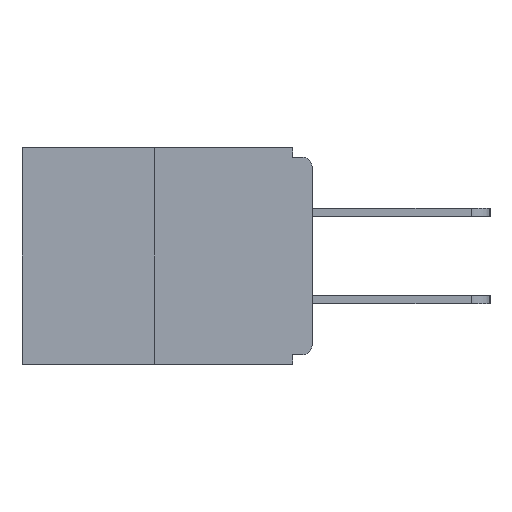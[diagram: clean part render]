
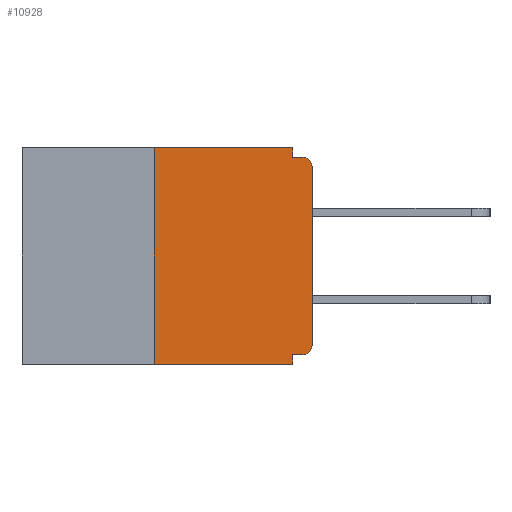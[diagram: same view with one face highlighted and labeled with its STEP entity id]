
A CAD part, left-side view. The second image highlights one B-rep face of the part: STEP entity #10928.
In plain terms, the highlighted planar face has unit normal (-1, 0, 0).
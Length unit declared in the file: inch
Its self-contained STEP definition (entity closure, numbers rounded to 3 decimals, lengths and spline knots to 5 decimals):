
#131 = EDGE_CURVE ( 'NONE', #7496, #12693, #7042, .T. ) ;
#219 = EDGE_CURVE ( 'NONE', #6645, #11678, #10148, .T. ) ;
#316 = CARTESIAN_POINT ( 'NONE',  ( 0., 0.46, 0. ) ) ;
#330 = CIRCLE ( 'NONE', #7711, 0.015 ) ;
#387 = CARTESIAN_POINT ( 'NONE',  ( 0., 0.031, -0.343 ) ) ;
#524 = PLANE ( 'NONE',  #10026 ) ;
#938 = ORIENTED_EDGE ( 'NONE', *, *, #5885, .T. ) ;
#1329 = LINE ( 'NONE', #316, #9888 ) ;
#1648 = CARTESIAN_POINT ( 'NONE',  ( 0., 0.25, 0. ) ) ;
#1830 = CARTESIAN_POINT ( 'NONE',  ( 0., 0.25, -0.343 ) ) ;
#2160 = VERTEX_POINT ( 'NONE', #387 ) ;
#2193 = DIRECTION ( 'NONE',  ( -1., 0., 0. ) ) ;
#2514 = AXIS2_PLACEMENT_3D ( 'NONE', #9028, #10268, #6293 ) ;
#2884 = VECTOR ( 'NONE', #3834, 39.37008 ) ;
#3396 = DIRECTION ( 'NONE',  ( 0., -1., 0. ) ) ;
#3625 = CARTESIAN_POINT ( 'NONE',  ( 0., 0.25, 0. ) ) ;
#3639 = EDGE_CURVE ( 'NONE', #6916, #2160, #11748, .T. ) ;
#3834 = DIRECTION ( 'NONE',  ( 0., 0., -1. ) ) ;
#3948 = VERTEX_POINT ( 'NONE', #9258 ) ;
#3983 = CARTESIAN_POINT ( 'NONE',  ( 0., 0.015, -0.328 ) ) ;
#4005 = ORIENTED_EDGE ( 'NONE', *, *, #7809, .T. ) ;
#4023 = CIRCLE ( 'NONE', #2514, 0.015 ) ;
#4101 = CARTESIAN_POINT ( 'NONE',  ( 0., 0., -0.328 ) ) ;
#4320 = CARTESIAN_POINT ( 'NONE',  ( 0., 0., -0.015 ) ) ;
#4569 = LINE ( 'NONE', #11820, #2884 ) ;
#4978 = EDGE_CURVE ( 'NONE', #11678, #2160, #4569, .T. ) ;
#5020 = DIRECTION ( 'NONE',  ( 0., 1., 0. ) ) ;
#5159 = VERTEX_POINT ( 'NONE', #3625 ) ;
#5363 = CARTESIAN_POINT ( 'NONE',  ( 0., 0.031, 0. ) ) ;
#5516 = DIRECTION ( 'NONE',  ( 1., 0., 0. ) ) ;
#5885 = EDGE_CURVE ( 'NONE', #3948, #9694, #330, .T. ) ;
#6252 = CARTESIAN_POINT ( 'NONE',  ( 0., 0.031, -0.328 ) ) ;
#6293 = DIRECTION ( 'NONE',  ( 0., 0., -1. ) ) ;
#6373 = CARTESIAN_POINT ( 'NONE',  ( 0., 0.031, 0. ) ) ;
#6432 = ORIENTED_EDGE ( 'NONE', *, *, #7724, .T. ) ;
#6645 = VERTEX_POINT ( 'NONE', #3983 ) ;
#6748 = LINE ( 'NONE', #4320, #11732 ) ;
#6855 = VECTOR ( 'NONE', #5020, 39.37008 ) ;
#6916 = VERTEX_POINT ( 'NONE', #1830 ) ;
#6959 = CARTESIAN_POINT ( 'NONE',  ( 0., 0.015, -0.015 ) ) ;
#7042 = LINE ( 'NONE', #6373, #10921 ) ;
#7084 = VECTOR ( 'NONE', #11537, 39.37008 ) ;
#7204 = VERTEX_POINT ( 'NONE', #12440 ) ;
#7321 = CARTESIAN_POINT ( 'NONE',  ( 0., 0., 0. ) ) ;
#7496 = VERTEX_POINT ( 'NONE', #5363 ) ;
#7711 = AXIS2_PLACEMENT_3D ( 'NONE', #9131, #2193, #9305 ) ;
#7724 = EDGE_CURVE ( 'NONE', #6645, #7204, #4023, .T. ) ;
#7809 = EDGE_CURVE ( 'NONE', #7204, #3948, #10874, .T. ) ;
#7840 = ORIENTED_EDGE ( 'NONE', *, *, #10229, .F. ) ;
#7892 = DIRECTION ( 'NONE',  ( 0., -1., 0. ) ) ;
#8022 = CARTESIAN_POINT ( 'NONE',  ( 0., 0.46, -0.343 ) ) ;
#8030 = EDGE_LOOP ( 'NONE', ( #11593, #9678, #10987, #10637, #8867, #6432, #4005, #938, #7840, #11430 ) ) ;
#8525 = CARTESIAN_POINT ( 'NONE',  ( 0., 0.031, -0.015 ) ) ;
#8867 = ORIENTED_EDGE ( 'NONE', *, *, #219, .F. ) ;
#9028 = CARTESIAN_POINT ( 'NONE',  ( 0., 0.015, -0.313 ) ) ;
#9131 = CARTESIAN_POINT ( 'NONE',  ( 0., 0.015, -0.03 ) ) ;
#9258 = CARTESIAN_POINT ( 'NONE',  ( 0., 0., -0.03 ) ) ;
#9305 = DIRECTION ( 'NONE',  ( 0., 0., -1. ) ) ;
#9399 = DIRECTION ( 'NONE',  ( 0., 0., -1. ) ) ;
#9501 = CARTESIAN_POINT ( 'NONE',  ( 0., 0.46, 0. ) ) ;
#9678 = ORIENTED_EDGE ( 'NONE', *, *, #9946, .F. ) ;
#9694 = VERTEX_POINT ( 'NONE', #6959 ) ;
#9888 = VECTOR ( 'NONE', #12142, 39.37008 ) ;
#9946 = EDGE_CURVE ( 'NONE', #6916, #5159, #10196, .T. ) ;
#10026 = AXIS2_PLACEMENT_3D ( 'NONE', #9501, #5516, #10561 ) ;
#10148 = LINE ( 'NONE', #4101, #6855 ) ;
#10196 = LINE ( 'NONE', #1648, #7084 ) ;
#10229 = EDGE_CURVE ( 'NONE', #12693, #9694, #6748, .T. ) ;
#10268 = DIRECTION ( 'NONE',  ( -1., 0., 0. ) ) ;
#10561 = DIRECTION ( 'NONE',  ( 0., 0., -1. ) ) ;
#10637 = ORIENTED_EDGE ( 'NONE', *, *, #4978, .F. ) ;
#10691 = VECTOR ( 'NONE', #7892, 39.37008 ) ;
#10874 = LINE ( 'NONE', #7321, #12265 ) ;
#10921 = VECTOR ( 'NONE', #9399, 39.37008 ) ;
#10928 = ADVANCED_FACE ( 'NONE', ( #11295 ), #524, .F. ) ;
#10987 = ORIENTED_EDGE ( 'NONE', *, *, #3639, .T. ) ;
#11189 = DIRECTION ( 'NONE',  ( 0., 0., 1. ) ) ;
#11295 = FACE_OUTER_BOUND ( 'NONE', #8030, .T. ) ;
#11430 = ORIENTED_EDGE ( 'NONE', *, *, #131, .F. ) ;
#11537 = DIRECTION ( 'NONE',  ( 0., 0., 1. ) ) ;
#11593 = ORIENTED_EDGE ( 'NONE', *, *, #11680, .F. ) ;
#11678 = VERTEX_POINT ( 'NONE', #6252 ) ;
#11680 = EDGE_CURVE ( 'NONE', #5159, #7496, #1329, .T. ) ;
#11732 = VECTOR ( 'NONE', #3396, 39.37008 ) ;
#11748 = LINE ( 'NONE', #8022, #10691 ) ;
#11820 = CARTESIAN_POINT ( 'NONE',  ( 0., 0.031, -0.343 ) ) ;
#12142 = DIRECTION ( 'NONE',  ( 0., -1., 0. ) ) ;
#12265 = VECTOR ( 'NONE', #11189, 39.37008 ) ;
#12440 = CARTESIAN_POINT ( 'NONE',  ( 0., 0., -0.313 ) ) ;
#12693 = VERTEX_POINT ( 'NONE', #8525 ) ;
